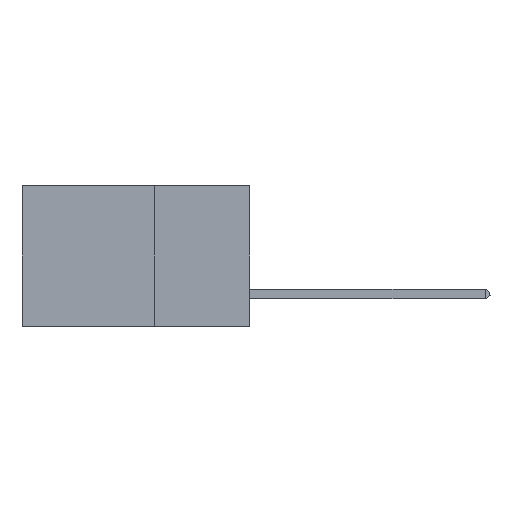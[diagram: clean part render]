
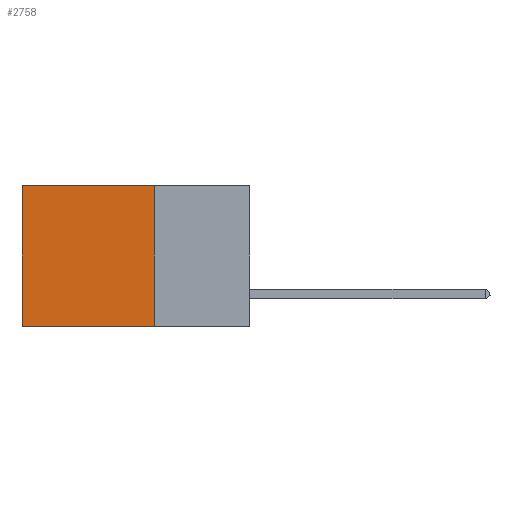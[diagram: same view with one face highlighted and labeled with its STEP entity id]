
A CAD part, left-side view. The second image highlights one B-rep face of the part: STEP entity #2758.
In plain terms, the highlighted planar face has unit normal (-1, 0, 0).
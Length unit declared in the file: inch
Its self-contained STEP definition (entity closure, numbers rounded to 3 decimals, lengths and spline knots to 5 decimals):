
#355 = VECTOR ( 'NONE', #13843, 39.37008 ) ;
#1848 = VERTEX_POINT ( 'NONE', #20743 ) ;
#2475 = EDGE_CURVE ( 'NONE', #12167, #18251, #6997, .T. ) ;
#2589 = CARTESIAN_POINT ( 'NONE',  ( 0.2875, 0.25, 0. ) ) ;
#2758 = ADVANCED_FACE ( 'NONE', ( #4577 ), #21087, .F. ) ;
#3170 = VERTEX_POINT ( 'NONE', #10811 ) ;
#3393 = CARTESIAN_POINT ( 'NONE',  ( 0.2875, 0.6, -0.37 ) ) ;
#3723 = VECTOR ( 'NONE', #18689, 39.37008 ) ;
#4061 = EDGE_CURVE ( 'NONE', #1848, #18251, #13294, .T. ) ;
#4577 = FACE_OUTER_BOUND ( 'NONE', #10968, .T. ) ;
#5267 = CARTESIAN_POINT ( 'NONE',  ( 0.2875, 0.6, 0. ) ) ;
#5718 = LINE ( 'NONE', #13776, #24145 ) ;
#6997 = LINE ( 'NONE', #5267, #355 ) ;
#9553 = ORIENTED_EDGE ( 'NONE', *, *, #4061, .F. ) ;
#10640 = LINE ( 'NONE', #18061, #3723 ) ;
#10811 = CARTESIAN_POINT ( 'NONE',  ( 0.2875, 0.25, 0. ) ) ;
#10968 = EDGE_LOOP ( 'NONE', ( #14147, #9553, #23151, #13686 ) ) ;
#12167 = VERTEX_POINT ( 'NONE', #15531 ) ;
#13294 = LINE ( 'NONE', #20958, #24021 ) ;
#13686 = ORIENTED_EDGE ( 'NONE', *, *, #24943, .T. ) ;
#13776 = CARTESIAN_POINT ( 'NONE',  ( 0.2875, 0.25, 0. ) ) ;
#13843 = DIRECTION ( 'NONE',  ( 0., 0., -1. ) ) ;
#14147 = ORIENTED_EDGE ( 'NONE', *, *, #2475, .T. ) ;
#14512 = AXIS2_PLACEMENT_3D ( 'NONE', #2589, #25091, #16903 ) ;
#15531 = CARTESIAN_POINT ( 'NONE',  ( 0.2875, 0.6, 0. ) ) ;
#16903 = DIRECTION ( 'NONE',  ( 0., 0., -1. ) ) ;
#18061 = CARTESIAN_POINT ( 'NONE',  ( 0.2875, 0.25, 0. ) ) ;
#18251 = VERTEX_POINT ( 'NONE', #3393 ) ;
#18689 = DIRECTION ( 'NONE',  ( 0., 1., 0. ) ) ;
#20743 = CARTESIAN_POINT ( 'NONE',  ( 0.2875, 0.25, -0.37 ) ) ;
#20958 = CARTESIAN_POINT ( 'NONE',  ( 0.2875, 0.25, -0.37 ) ) ;
#21087 = PLANE ( 'NONE',  #14512 ) ;
#21995 = EDGE_CURVE ( 'NONE', #3170, #1848, #5718, .T. ) ;
#23151 = ORIENTED_EDGE ( 'NONE', *, *, #21995, .F. ) ;
#24021 = VECTOR ( 'NONE', #25237, 39.37008 ) ;
#24145 = VECTOR ( 'NONE', #25845, 39.37008 ) ;
#24943 = EDGE_CURVE ( 'NONE', #3170, #12167, #10640, .T. ) ;
#25091 = DIRECTION ( 'NONE',  ( 1., 0., 0. ) ) ;
#25237 = DIRECTION ( 'NONE',  ( 0., 1., 0. ) ) ;
#25845 = DIRECTION ( 'NONE',  ( 0., 0., -1. ) ) ;
